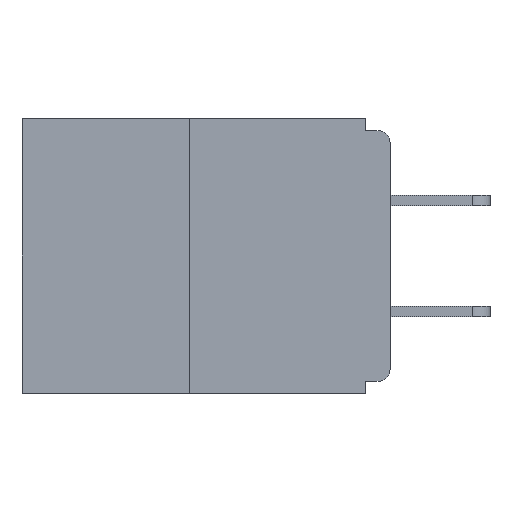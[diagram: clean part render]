
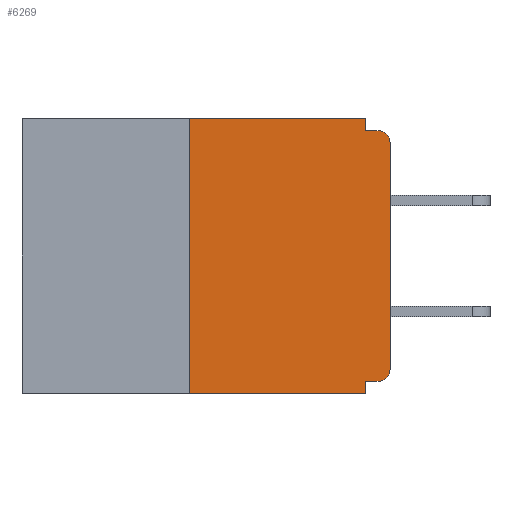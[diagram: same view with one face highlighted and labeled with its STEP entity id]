
A CAD part, left-side view. The second image highlights one B-rep face of the part: STEP entity #6269.
In plain terms, the highlighted planar face has unit normal (-1, 0, 0).
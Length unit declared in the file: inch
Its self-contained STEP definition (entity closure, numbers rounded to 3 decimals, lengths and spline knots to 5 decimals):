
#72 = CARTESIAN_POINT ( 'NONE',  ( 0., 0.015, -0.328 ) ) ;
#99 = CARTESIAN_POINT ( 'NONE',  ( 0., 0., 0. ) ) ;
#445 = DIRECTION ( 'NONE',  ( 0., -1., 0. ) ) ;
#484 = AXIS2_PLACEMENT_3D ( 'NONE', #1169, #5350, #2007 ) ;
#563 = DIRECTION ( 'NONE',  ( 0., 0., -1. ) ) ;
#677 = DIRECTION ( 'NONE',  ( 0., -1., 0. ) ) ;
#995 = VERTEX_POINT ( 'NONE', #9827 ) ;
#1070 = CARTESIAN_POINT ( 'NONE',  ( 0., 0.031, -0.343 ) ) ;
#1099 = LINE ( 'NONE', #5015, #9936 ) ;
#1169 = CARTESIAN_POINT ( 'NONE',  ( 0., 0.46, 0. ) ) ;
#1188 = DIRECTION ( 'NONE',  ( 0., 0., 1. ) ) ;
#1267 = LINE ( 'NONE', #9471, #5418 ) ;
#1372 = CARTESIAN_POINT ( 'NONE',  ( 0., 0.46, 0. ) ) ;
#1689 = VERTEX_POINT ( 'NONE', #9029 ) ;
#1690 = EDGE_CURVE ( 'NONE', #5592, #6528, #5792, .T. ) ;
#1692 = VERTEX_POINT ( 'NONE', #72 ) ;
#1698 = DIRECTION ( 'NONE',  ( 0., 1., 0. ) ) ;
#1795 = PLANE ( 'NONE',  #484 ) ;
#1826 = VERTEX_POINT ( 'NONE', #1070 ) ;
#2007 = DIRECTION ( 'NONE',  ( 0., 0., -1. ) ) ;
#2254 = VECTOR ( 'NONE', #9917, 39.37008 ) ;
#2433 = DIRECTION ( 'NONE',  ( 0., 0., -1. ) ) ;
#2460 = EDGE_CURVE ( 'NONE', #8703, #4260, #3320, .T. ) ;
#2534 = DIRECTION ( 'NONE',  ( -1., 0., 0. ) ) ;
#2761 = EDGE_CURVE ( 'NONE', #1692, #995, #1099, .T. ) ;
#2849 = ORIENTED_EDGE ( 'NONE', *, *, #8953, .T. ) ;
#3004 = CARTESIAN_POINT ( 'NONE',  ( 0., 0.031, 0. ) ) ;
#3137 = EDGE_CURVE ( 'NONE', #6349, #5592, #8377, .T. ) ;
#3320 = LINE ( 'NONE', #1372, #6047 ) ;
#3645 = CARTESIAN_POINT ( 'NONE',  ( 0., 0.25, 0. ) ) ;
#3755 = ORIENTED_EDGE ( 'NONE', *, *, #9135, .F. ) ;
#4086 = ORIENTED_EDGE ( 'NONE', *, *, #2761, .F. ) ;
#4168 = LINE ( 'NONE', #6605, #10539 ) ;
#4213 = CARTESIAN_POINT ( 'NONE',  ( 0., 0.015, -0.015 ) ) ;
#4260 = VERTEX_POINT ( 'NONE', #3004 ) ;
#4336 = ORIENTED_EDGE ( 'NONE', *, *, #4787, .F. ) ;
#4422 = CARTESIAN_POINT ( 'NONE',  ( 0., 0., -0.03 ) ) ;
#4787 = EDGE_CURVE ( 'NONE', #4260, #5045, #6312, .T. ) ;
#5015 = CARTESIAN_POINT ( 'NONE',  ( 0., 0., -0.328 ) ) ;
#5045 = VERTEX_POINT ( 'NONE', #10351 ) ;
#5350 = DIRECTION ( 'NONE',  ( 1., 0., 0. ) ) ;
#5418 = VECTOR ( 'NONE', #1188, 39.37008 ) ;
#5539 = ORIENTED_EDGE ( 'NONE', *, *, #10503, .F. ) ;
#5592 = VERTEX_POINT ( 'NONE', #4422 ) ;
#5616 = FACE_OUTER_BOUND ( 'NONE', #9572, .T. ) ;
#5727 = CARTESIAN_POINT ( 'NONE',  ( 0., 0.46, -0.343 ) ) ;
#5741 = DIRECTION ( 'NONE',  ( 0., 0., -1. ) ) ;
#5792 = CIRCLE ( 'NONE', #10755, 0.015 ) ;
#5807 = DIRECTION ( 'NONE',  ( 0., -1., 0. ) ) ;
#5857 = CARTESIAN_POINT ( 'NONE',  ( 0., 0.015, -0.03 ) ) ;
#6047 = VECTOR ( 'NONE', #445, 39.37008 ) ;
#6206 = CIRCLE ( 'NONE', #8979, 0.015 ) ;
#6269 = ADVANCED_FACE ( 'NONE', ( #5616 ), #1795, .F. ) ;
#6312 = LINE ( 'NONE', #9685, #10237 ) ;
#6349 = VERTEX_POINT ( 'NONE', #7755 ) ;
#6467 = LINE ( 'NONE', #10496, #6854 ) ;
#6528 = VERTEX_POINT ( 'NONE', #4213 ) ;
#6605 = CARTESIAN_POINT ( 'NONE',  ( 0., 0., -0.015 ) ) ;
#6854 = VECTOR ( 'NONE', #9741, 39.37008 ) ;
#7379 = CARTESIAN_POINT ( 'NONE',  ( 0., 0.015, -0.313 ) ) ;
#7460 = DIRECTION ( 'NONE',  ( -1., 0., 0. ) ) ;
#7755 = CARTESIAN_POINT ( 'NONE',  ( 0., 0., -0.313 ) ) ;
#8234 = ORIENTED_EDGE ( 'NONE', *, *, #2460, .F. ) ;
#8377 = LINE ( 'NONE', #99, #2254 ) ;
#8432 = VECTOR ( 'NONE', #677, 39.37008 ) ;
#8561 = LINE ( 'NONE', #5727, #8432 ) ;
#8703 = VERTEX_POINT ( 'NONE', #3645 ) ;
#8953 = EDGE_CURVE ( 'NONE', #1689, #1826, #8561, .T. ) ;
#8979 = AXIS2_PLACEMENT_3D ( 'NONE', #7379, #2534, #2433 ) ;
#9029 = CARTESIAN_POINT ( 'NONE',  ( 0., 0.25, -0.343 ) ) ;
#9122 = ORIENTED_EDGE ( 'NONE', *, *, #1690, .T. ) ;
#9135 = EDGE_CURVE ( 'NONE', #5045, #6528, #4168, .T. ) ;
#9471 = CARTESIAN_POINT ( 'NONE',  ( 0., 0.25, 0. ) ) ;
#9564 = EDGE_CURVE ( 'NONE', #995, #1826, #6467, .T. ) ;
#9572 = EDGE_LOOP ( 'NONE', ( #8234, #5539, #2849, #9905, #4086, #10691, #10620, #9122, #3755, #4336 ) ) ;
#9679 = EDGE_CURVE ( 'NONE', #1692, #6349, #6206, .T. ) ;
#9685 = CARTESIAN_POINT ( 'NONE',  ( 0., 0.031, 0. ) ) ;
#9741 = DIRECTION ( 'NONE',  ( 0., 0., -1. ) ) ;
#9827 = CARTESIAN_POINT ( 'NONE',  ( 0., 0.031, -0.328 ) ) ;
#9905 = ORIENTED_EDGE ( 'NONE', *, *, #9564, .F. ) ;
#9917 = DIRECTION ( 'NONE',  ( 0., 0., 1. ) ) ;
#9936 = VECTOR ( 'NONE', #1698, 39.37008 ) ;
#10237 = VECTOR ( 'NONE', #563, 39.37008 ) ;
#10351 = CARTESIAN_POINT ( 'NONE',  ( 0., 0.031, -0.015 ) ) ;
#10496 = CARTESIAN_POINT ( 'NONE',  ( 0., 0.031, -0.343 ) ) ;
#10503 = EDGE_CURVE ( 'NONE', #1689, #8703, #1267, .T. ) ;
#10539 = VECTOR ( 'NONE', #5807, 39.37008 ) ;
#10620 = ORIENTED_EDGE ( 'NONE', *, *, #3137, .T. ) ;
#10691 = ORIENTED_EDGE ( 'NONE', *, *, #9679, .T. ) ;
#10755 = AXIS2_PLACEMENT_3D ( 'NONE', #5857, #7460, #5741 ) ;
